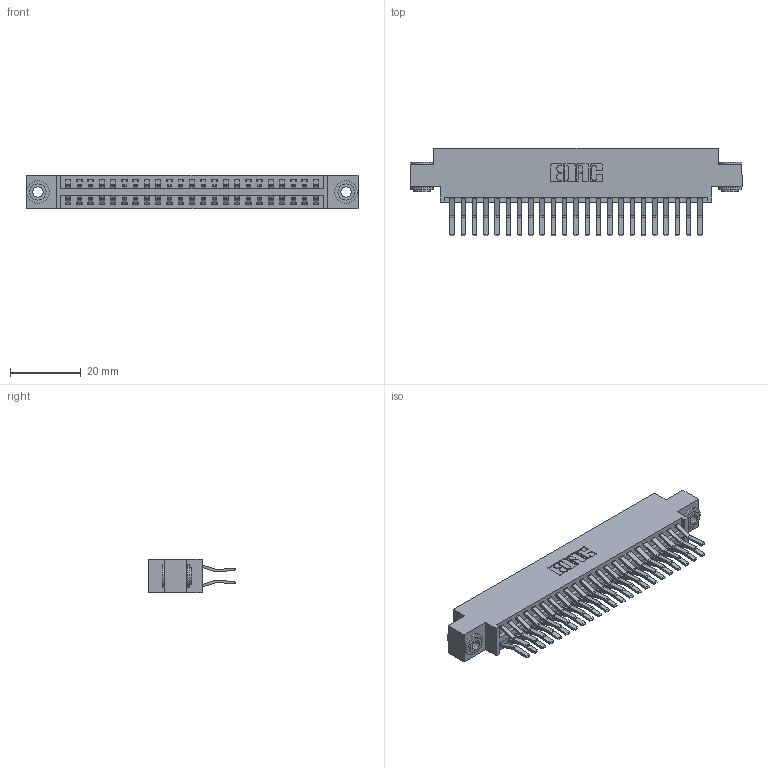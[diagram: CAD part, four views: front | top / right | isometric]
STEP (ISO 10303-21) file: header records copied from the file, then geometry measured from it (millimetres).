
FILE_DESCRIPTION (( 'STEP AP203' ), '1' );
FILE_NAME ('346-046-560-803.STEP', '2022-05-20T20:46:30', ( '' ), ( '' ), 'SwSTEP 2.0', 'SolidWorks 2020', '' );
FILE_SCHEMA (( 'CONFIG_CONTROL_DESIGN' ));
Length unit declared in the file: inch
Products named in the file (4): 346 Part_0.170 Offset - 0.156 Dia-TH; 346-046-560-803; 345-292-001_560 Tail; 345-250-002_345-250-002-102
Assembly tree (49 placements, depth 2):
  346-046-560-803
    346 Part_0.170 Offset - 0.156 Dia-TH
    345-292-001_560 Tail  x46
    345-250-002_345-250-002-102  x2
Bounding box: 93.6 x 24.78 x 9.4 mm (x, y, z)
Volume: 9127.7 mm3; surface area: 13480.8 mm2
Topology: 49 solids, 49 shells, 2662 faces, 7859 edges, 5174 vertices
Faces by surface type: plane 1714, cylinder 940, cone 8
Entity records: 18854 total; most frequent: CARTESIAN_POINT 3117, ORIENTED_EDGE 3042, DIRECTION 2831, EDGE_CURVE 1521, VECTOR 1269, LINE 1269, VERTEX_POINT 1010, AXIS2_PLACEMENT_3D 781
